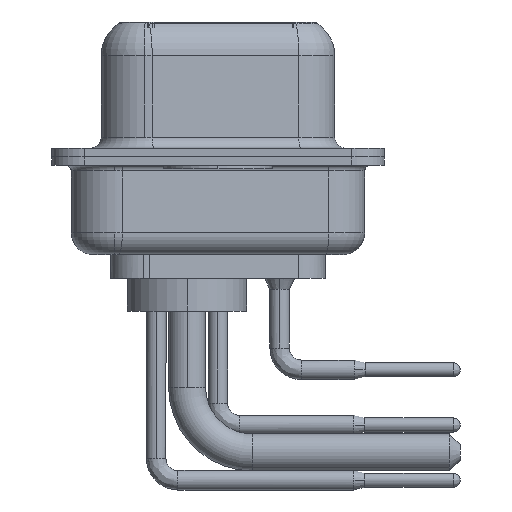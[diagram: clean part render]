
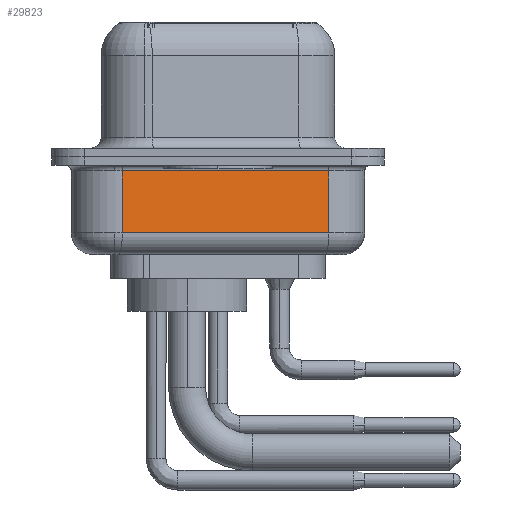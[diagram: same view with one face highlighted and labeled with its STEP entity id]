
A CAD part, left-side view. The second image highlights one B-rep face of the part: STEP entity #29823.
In plain terms, the highlighted planar face has unit normal (-0.985, -0.174, 0).
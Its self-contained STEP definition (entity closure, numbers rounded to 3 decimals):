
#282 = VERTEX_POINT ( 'NONE', #24911 ) ;
#495 = DIRECTION ( 'NONE',  ( 0., 0., 1. ) ) ;
#817 = ORIENTED_EDGE ( 'NONE', *, *, #6427, .F. ) ;
#1462 = LINE ( 'NONE', #10967, #5478 ) ;
#1938 = VERTEX_POINT ( 'NONE', #30341 ) ;
#1999 = DIRECTION ( 'NONE',  ( 0.985, 0.174, 0. ) ) ;
#2329 = CARTESIAN_POINT ( 'NONE',  ( 4.605, -5.097, -0.65 ) ) ;
#4403 = EDGE_CURVE ( 'NONE', #282, #5423, #20422, .T. ) ;
#5423 = VERTEX_POINT ( 'NONE', #2329 ) ;
#5478 = VECTOR ( 'NONE', #18854, 1000. ) ;
#6427 = EDGE_CURVE ( 'NONE', #1938, #17003, #21493, .T. ) ;
#7195 = ORIENTED_EDGE ( 'NONE', *, *, #4403, .T. ) ;
#7516 = CARTESIAN_POINT ( 'NONE',  ( 2.93, 4.403, -4.5 ) ) ;
#7736 = ORIENTED_EDGE ( 'NONE', *, *, #22848, .T. ) ;
#8617 = ORIENTED_EDGE ( 'NONE', *, *, #27486, .T. ) ;
#10967 = CARTESIAN_POINT ( 'NONE',  ( 2.93, 4.403, -0.65 ) ) ;
#12030 = AXIS2_PLACEMENT_3D ( 'NONE', #23309, #1999, #15865 ) ;
#13671 = EDGE_LOOP ( 'NONE', ( #817, #7736, #7195, #8617 ) ) ;
#13839 = FACE_OUTER_BOUND ( 'NONE', #13671, .T. ) ;
#15865 = DIRECTION ( 'NONE',  ( -0.174, 0.985, 0. ) ) ;
#17003 = VERTEX_POINT ( 'NONE', #23281 ) ;
#17947 = CARTESIAN_POINT ( 'NONE',  ( 4.605, -5.097, -4.5 ) ) ;
#18854 = DIRECTION ( 'NONE',  ( -0.174, 0.985, 0. ) ) ;
#19771 = VECTOR ( 'NONE', #23234, 1000. ) ;
#20422 = LINE ( 'NONE', #17947, #30031 ) ;
#20736 = CARTESIAN_POINT ( 'NONE',  ( 2.93, 4.403, -3.5 ) ) ;
#21471 = VECTOR ( 'NONE', #495, 1000. ) ;
#21493 = LINE ( 'NONE', #7516, #21471 ) ;
#22848 = EDGE_CURVE ( 'NONE', #1938, #282, #30072, .T. ) ;
#23234 = DIRECTION ( 'NONE',  ( 0.174, -0.985, 0. ) ) ;
#23281 = CARTESIAN_POINT ( 'NONE',  ( 2.93, 4.403, -0.65 ) ) ;
#23309 = CARTESIAN_POINT ( 'NONE',  ( 2.93, 4.403, -4.5 ) ) ;
#24911 = CARTESIAN_POINT ( 'NONE',  ( 4.605, -5.097, -3.5 ) ) ;
#25958 = PLANE ( 'NONE',  #12030 ) ;
#27486 = EDGE_CURVE ( 'NONE', #5423, #17003, #1462, .T. ) ;
#29435 = DIRECTION ( 'NONE',  ( 0., 0., 1. ) ) ;
#29823 = ADVANCED_FACE ( 'NONE', ( #13839 ), #25958, .F. ) ;
#30031 = VECTOR ( 'NONE', #29435, 1000. ) ;
#30072 = LINE ( 'NONE', #20736, #19771 ) ;
#30341 = CARTESIAN_POINT ( 'NONE',  ( 2.93, 4.403, -3.5 ) ) ;
